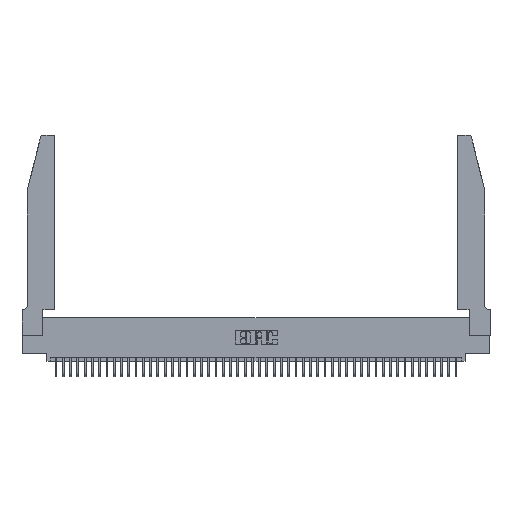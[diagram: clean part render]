
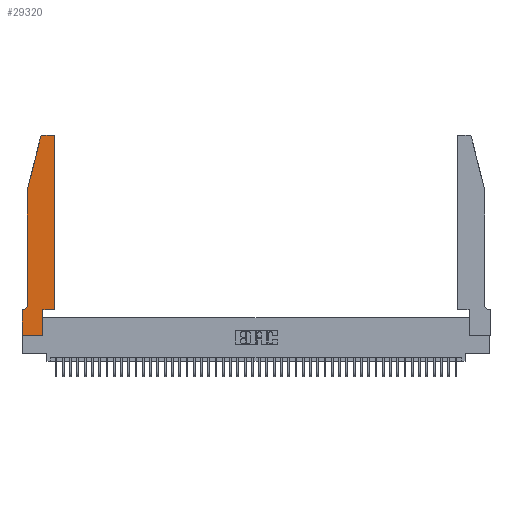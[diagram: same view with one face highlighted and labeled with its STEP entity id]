
A CAD part, top view. The second image highlights one B-rep face of the part: STEP entity #29320.
In plain terms, the highlighted planar face has unit normal (0, 0, 1).
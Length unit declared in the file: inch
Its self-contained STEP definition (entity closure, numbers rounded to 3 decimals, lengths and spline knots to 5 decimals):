
#155 = DIRECTION ( 'NONE',  ( 0., 0., 1. ) ) ;
#864 = DIRECTION ( 'NONE',  ( 0., 0., 1. ) ) ;
#956 = CARTESIAN_POINT ( 'NONE',  ( 0.4505, 2.72, 0.37 ) ) ;
#986 = ORIENTED_EDGE ( 'NONE', *, *, #25079, .T. ) ;
#2202 = DIRECTION ( 'NONE',  ( -1., 0., 0. ) ) ;
#2270 = EDGE_CURVE ( 'NONE', #5277, #13959, #47609, .T. ) ;
#2917 = LINE ( 'NONE', #19054, #41761 ) ;
#3473 = LINE ( 'NONE', #24917, #23695 ) ;
#3514 = CARTESIAN_POINT ( 'NONE',  ( 0., 0., 0.37 ) ) ;
#3960 = VERTEX_POINT ( 'NONE', #6101 ) ;
#4322 = CARTESIAN_POINT ( 'NONE',  ( 0., 0.35, 0.37 ) ) ;
#4866 = VERTEX_POINT ( 'NONE', #18837 ) ;
#5176 = VECTOR ( 'NONE', #12807, 39.37008 ) ;
#5259 = ORIENTED_EDGE ( 'NONE', *, *, #18916, .T. ) ;
#5277 = VERTEX_POINT ( 'NONE', #6731 ) ;
#5441 = DIRECTION ( 'NONE',  ( 0., -1., 0. ) ) ;
#6101 = CARTESIAN_POINT ( 'NONE',  ( 0.0755, 0.42, 0.37 ) ) ;
#6295 = VECTOR ( 'NONE', #48281, 39.37008 ) ;
#6731 = CARTESIAN_POINT ( 'NONE',  ( 0.0055, 0.35, 0.37 ) ) ;
#6869 = CARTESIAN_POINT ( 'NONE',  ( 0.284, 2.72, 0.37 ) ) ;
#7019 = DIRECTION ( 'NONE',  ( 0., 1., 0. ) ) ;
#7562 = CARTESIAN_POINT ( 'NONE',  ( 0.0055, 0.42, 0.37 ) ) ;
#8616 = CARTESIAN_POINT ( 'NONE',  ( 0.284, 2.75, 0.37 ) ) ;
#8751 = ORIENTED_EDGE ( 'NONE', *, *, #39210, .T. ) ;
#9192 = ORIENTED_EDGE ( 'NONE', *, *, #2270, .T. ) ;
#10309 = VECTOR ( 'NONE', #5441, 39.37008 ) ;
#10461 = ORIENTED_EDGE ( 'NONE', *, *, #23270, .T. ) ;
#10475 = EDGE_CURVE ( 'NONE', #4866, #11860, #3473, .T. ) ;
#10617 = CARTESIAN_POINT ( 'NONE',  ( 0.0755, 2., 0.37 ) ) ;
#10705 = DIRECTION ( 'NONE',  ( 1., 0., 0. ) ) ;
#10814 = FACE_OUTER_BOUND ( 'NONE', #12409, .T. ) ;
#11401 = DIRECTION ( 'NONE',  ( -1., 0., 0. ) ) ;
#11516 = LINE ( 'NONE', #20572, #10309 ) ;
#11860 = VERTEX_POINT ( 'NONE', #8616 ) ;
#12238 = EDGE_CURVE ( 'NONE', #3960, #5277, #21255, .T. ) ;
#12409 = EDGE_LOOP ( 'NONE', ( #27168, #986, #36146, #8751, #36476, #9192, #40630, #29404, #14713, #10461, #5259, #25933 ) ) ;
#12807 = DIRECTION ( 'NONE',  ( 1., 0., 0. ) ) ;
#13959 = VERTEX_POINT ( 'NONE', #4322 ) ;
#14637 = VECTOR ( 'NONE', #28461, 39.37008 ) ;
#14713 = ORIENTED_EDGE ( 'NONE', *, *, #21378, .T. ) ;
#14765 = AXIS2_PLACEMENT_3D ( 'NONE', #6869, #33158, #10705 ) ;
#17908 = VECTOR ( 'NONE', #18242, 39.37008 ) ;
#18113 = DIRECTION ( 'NONE',  ( -0.239, -0.971, 0. ) ) ;
#18242 = DIRECTION ( 'NONE',  ( -1., 0., 0. ) ) ;
#18837 = CARTESIAN_POINT ( 'NONE',  ( 0.4205, 2.75, 0.37 ) ) ;
#18916 = EDGE_CURVE ( 'NONE', #47164, #26812, #2917, .T. ) ;
#19054 = CARTESIAN_POINT ( 'NONE',  ( 0.4505, 0.35, 0.37 ) ) ;
#20072 = LINE ( 'NONE', #10617, #48586 ) ;
#20144 = EDGE_CURVE ( 'NONE', #32178, #26651, #20072, .T. ) ;
#20449 = CARTESIAN_POINT ( 'NONE',  ( 0.4505, 0.35, 0.37 ) ) ;
#20572 = CARTESIAN_POINT ( 'NONE',  ( 0.0755, 2., 0.37 ) ) ;
#21255 = CIRCLE ( 'NONE', #35348, 0.07 ) ;
#21378 = EDGE_CURVE ( 'NONE', #42777, #32844, #44382, .T. ) ;
#22657 = CARTESIAN_POINT ( 'NONE',  ( 0.25487, 2.72718, 0.37 ) ) ;
#22853 = EDGE_CURVE ( 'NONE', #26812, #4866, #39856, .T. ) ;
#23270 = EDGE_CURVE ( 'NONE', #32844, #47164, #36281, .T. ) ;
#23642 = CARTESIAN_POINT ( 'NONE',  ( 0.4205, 2.72, 0.37 ) ) ;
#23695 = VECTOR ( 'NONE', #2202, 39.37008 ) ;
#24546 = CARTESIAN_POINT ( 'NONE',  ( 0., 0., 0.37 ) ) ;
#24917 = CARTESIAN_POINT ( 'NONE',  ( 0.2605, 2.75, 0.37 ) ) ;
#25079 = EDGE_CURVE ( 'NONE', #11860, #32178, #36113, .T. ) ;
#25816 = LINE ( 'NONE', #24546, #14637 ) ;
#25933 = ORIENTED_EDGE ( 'NONE', *, *, #22853, .T. ) ;
#26593 = DIRECTION ( 'NONE',  ( 0., 1., 0. ) ) ;
#26651 = VERTEX_POINT ( 'NONE', #30560 ) ;
#26666 = DIRECTION ( 'NONE',  ( 1., 0., 0. ) ) ;
#26812 = VERTEX_POINT ( 'NONE', #956 ) ;
#27168 = ORIENTED_EDGE ( 'NONE', *, *, #10475, .T. ) ;
#27385 = DIRECTION ( 'NONE',  ( 1., 0., 0. ) ) ;
#27792 = CARTESIAN_POINT ( 'NONE',  ( 0., 0., 0.37 ) ) ;
#28461 = DIRECTION ( 'NONE',  ( 0., -1., 0. ) ) ;
#28723 = AXIS2_PLACEMENT_3D ( 'NONE', #30245, #155, #26666 ) ;
#29320 = ADVANCED_FACE ( 'NONE', ( #10814 ), #45158, .T. ) ;
#29404 = ORIENTED_EDGE ( 'NONE', *, *, #31414, .T. ) ;
#29623 = CARTESIAN_POINT ( 'NONE',  ( 0.2865, 0.35, 0.37 ) ) ;
#30245 = CARTESIAN_POINT ( 'NONE',  ( 0., 0.35, 0.37 ) ) ;
#30560 = CARTESIAN_POINT ( 'NONE',  ( 0.0755, 2., 0.37 ) ) ;
#31414 = EDGE_CURVE ( 'NONE', #45759, #42777, #47419, .T. ) ;
#32178 = VERTEX_POINT ( 'NONE', #22657 ) ;
#32546 = EDGE_CURVE ( 'NONE', #13959, #45759, #25816, .T. ) ;
#32844 = VERTEX_POINT ( 'NONE', #38360 ) ;
#33158 = DIRECTION ( 'NONE',  ( 0., 0., 1. ) ) ;
#33840 = DIRECTION ( 'NONE',  ( 0., 0., -1. ) ) ;
#35348 = AXIS2_PLACEMENT_3D ( 'NONE', #7562, #33840, #11401 ) ;
#36113 = CIRCLE ( 'NONE', #14765, 0.03 ) ;
#36146 = ORIENTED_EDGE ( 'NONE', *, *, #20144, .T. ) ;
#36207 = CARTESIAN_POINT ( 'NONE',  ( 0.2865, 0., 0.37 ) ) ;
#36281 = LINE ( 'NONE', #44537, #6295 ) ;
#36476 = ORIENTED_EDGE ( 'NONE', *, *, #12238, .T. ) ;
#38360 = CARTESIAN_POINT ( 'NONE',  ( 0.2865, 0.35, 0.37 ) ) ;
#39210 = EDGE_CURVE ( 'NONE', #26651, #3960, #11516, .T. ) ;
#39856 = CIRCLE ( 'NONE', #45625, 0.03 ) ;
#40630 = ORIENTED_EDGE ( 'NONE', *, *, #32546, .T. ) ;
#41761 = VECTOR ( 'NONE', #26593, 39.37008 ) ;
#42777 = VERTEX_POINT ( 'NONE', #36207 ) ;
#44282 = CARTESIAN_POINT ( 'NONE',  ( 0.0755, 0.35, 0.37 ) ) ;
#44382 = LINE ( 'NONE', #29623, #45565 ) ;
#44537 = CARTESIAN_POINT ( 'NONE',  ( 0.4505, 0.35, 0.37 ) ) ;
#45158 = PLANE ( 'NONE',  #28723 ) ;
#45565 = VECTOR ( 'NONE', #7019, 39.37008 ) ;
#45625 = AXIS2_PLACEMENT_3D ( 'NONE', #23642, #864, #27385 ) ;
#45759 = VERTEX_POINT ( 'NONE', #3514 ) ;
#47164 = VERTEX_POINT ( 'NONE', #20449 ) ;
#47419 = LINE ( 'NONE', #27792, #5176 ) ;
#47609 = LINE ( 'NONE', #44282, #17908 ) ;
#48281 = DIRECTION ( 'NONE',  ( 1., 0., 0. ) ) ;
#48586 = VECTOR ( 'NONE', #18113, 39.37008 ) ;
